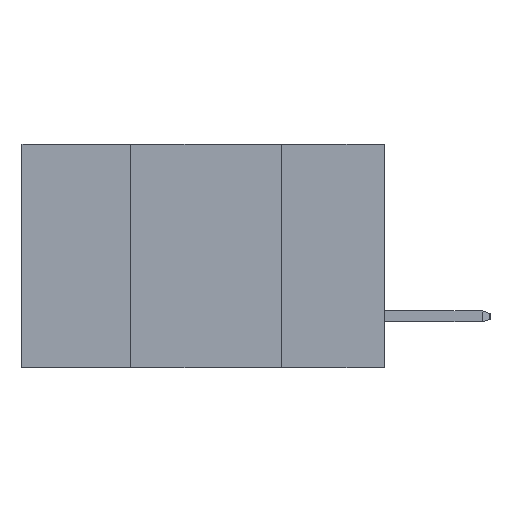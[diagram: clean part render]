
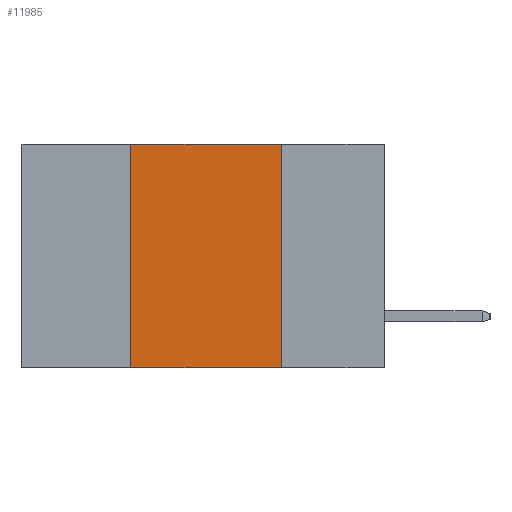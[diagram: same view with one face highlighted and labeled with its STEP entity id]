
A CAD part, left-side view. The second image highlights one B-rep face of the part: STEP entity #11985.
In plain terms, the highlighted planar face has unit normal (-1, 0, 0).
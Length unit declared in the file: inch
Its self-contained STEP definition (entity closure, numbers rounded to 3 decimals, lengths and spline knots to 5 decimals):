
#6 = VERTEX_POINT ( 'NONE', #6340 ) ;
#93 = ORIENTED_EDGE ( 'NONE', *, *, #5939, .F. ) ;
#106 = CARTESIAN_POINT ( 'NONE',  ( 0., 0.6, 0. ) ) ;
#1350 = VECTOR ( 'NONE', #11654, 39.37008 ) ;
#1536 = VECTOR ( 'NONE', #5367, 39.37008 ) ;
#1573 = DIRECTION ( 'NONE',  ( 0., 0., -1. ) ) ;
#2058 = VECTOR ( 'NONE', #7772, 39.37008 ) ;
#2076 = EDGE_LOOP ( 'NONE', ( #6116, #93, #7623, #12648 ) ) ;
#2236 = FACE_OUTER_BOUND ( 'NONE', #2076, .T. ) ;
#2716 = CARTESIAN_POINT ( 'NONE',  ( 0., 0.17, 0. ) ) ;
#3572 = LINE ( 'NONE', #9292, #9983 ) ;
#3616 = CARTESIAN_POINT ( 'NONE',  ( 0., 0.42, 0. ) ) ;
#5266 = CARTESIAN_POINT ( 'NONE',  ( 0., 0.17, -0.37 ) ) ;
#5367 = DIRECTION ( 'NONE',  ( 0., 0., -1. ) ) ;
#5939 = EDGE_CURVE ( 'NONE', #10225, #6, #3572, .T. ) ;
#6116 = ORIENTED_EDGE ( 'NONE', *, *, #14087, .F. ) ;
#6340 = CARTESIAN_POINT ( 'NONE',  ( 0., 0.17, 0. ) ) ;
#7623 = ORIENTED_EDGE ( 'NONE', *, *, #13243, .F. ) ;
#7772 = DIRECTION ( 'NONE',  ( 0., -1., 0. ) ) ;
#8205 = LINE ( 'NONE', #2716, #1536 ) ;
#9059 = DIRECTION ( 'NONE',  ( 0., -1., 0. ) ) ;
#9292 = CARTESIAN_POINT ( 'NONE',  ( 0., 0.6, 0. ) ) ;
#9482 = DIRECTION ( 'NONE',  ( 1., 0., 0. ) ) ;
#9983 = VECTOR ( 'NONE', #9059, 39.37008 ) ;
#10225 = VERTEX_POINT ( 'NONE', #3616 ) ;
#10420 = CARTESIAN_POINT ( 'NONE',  ( 0., 0.42, 0. ) ) ;
#10959 = CARTESIAN_POINT ( 'NONE',  ( 0., 0.42, -0.37 ) ) ;
#11654 = DIRECTION ( 'NONE',  ( 0., 0., 1. ) ) ;
#11927 = AXIS2_PLACEMENT_3D ( 'NONE', #106, #9482, #1573 ) ;
#11985 = ADVANCED_FACE ( 'NONE', ( #2236 ), #15647, .F. ) ;
#12339 = LINE ( 'NONE', #15213, #2058 ) ;
#12437 = EDGE_CURVE ( 'NONE', #12818, #12466, #12339, .T. ) ;
#12466 = VERTEX_POINT ( 'NONE', #5266 ) ;
#12648 = ORIENTED_EDGE ( 'NONE', *, *, #12437, .T. ) ;
#12818 = VERTEX_POINT ( 'NONE', #10959 ) ;
#13243 = EDGE_CURVE ( 'NONE', #12818, #10225, #15037, .T. ) ;
#14087 = EDGE_CURVE ( 'NONE', #6, #12466, #8205, .T. ) ;
#15037 = LINE ( 'NONE', #10420, #1350 ) ;
#15213 = CARTESIAN_POINT ( 'NONE',  ( 0., 0.6, -0.37 ) ) ;
#15647 = PLANE ( 'NONE',  #11927 ) ;
